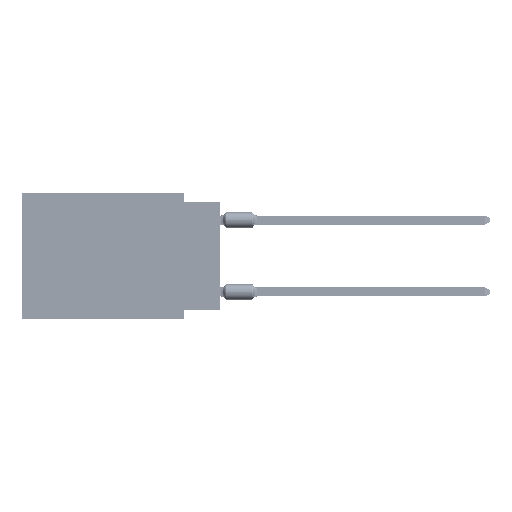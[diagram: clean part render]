
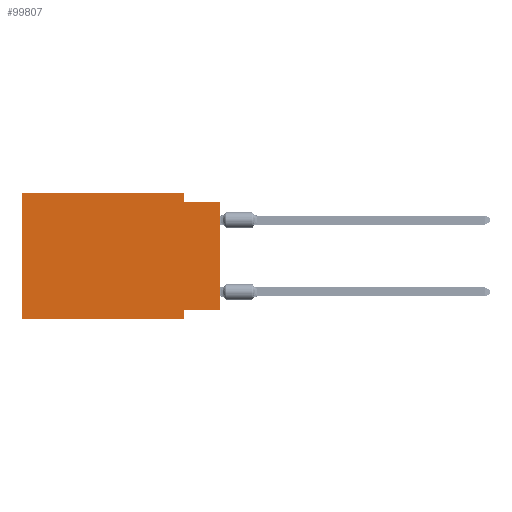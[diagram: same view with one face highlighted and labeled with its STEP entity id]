
A CAD part, left-side view. The second image highlights one B-rep face of the part: STEP entity #99807.
In plain terms, the highlighted planar face has unit normal (-1, 0, 0).
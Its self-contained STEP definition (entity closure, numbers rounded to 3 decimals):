
#3173 = VERTEX_POINT ( 'NONE', #75781 ) ;
#4792 = VERTEX_POINT ( 'NONE', #20576 ) ;
#7145 = EDGE_CURVE ( 'NONE', #107195, #94920, #32099, .T. ) ;
#7536 = AXIS2_PLACEMENT_3D ( 'NONE', #93989, #10364, #17118 ) ;
#9249 = VECTOR ( 'NONE', #37424, 1000. ) ;
#10364 = DIRECTION ( 'NONE',  ( 1., 0., 0. ) ) ;
#14214 = VECTOR ( 'NONE', #97078, 1000. ) ;
#14632 = CARTESIAN_POINT ( 'NONE',  ( 0., 0., -8.255 ) ) ;
#15207 = CARTESIAN_POINT ( 'NONE',  ( 0., 13.97, 0. ) ) ;
#15430 = EDGE_CURVE ( 'NONE', #4792, #97999, #85093, .T. ) ;
#17118 = DIRECTION ( 'NONE',  ( 0., 0., -1. ) ) ;
#20576 = CARTESIAN_POINT ( 'NONE',  ( 0., 2.54, 0. ) ) ;
#21849 = ORIENTED_EDGE ( 'NONE', *, *, #43082, .F. ) ;
#23670 = DIRECTION ( 'NONE',  ( 0., 0., 1. ) ) ;
#25764 = VECTOR ( 'NONE', #55518, 1000. ) ;
#26740 = LINE ( 'NONE', #52032, #101322 ) ;
#28451 = CARTESIAN_POINT ( 'NONE',  ( 0., 2.54, -8.89 ) ) ;
#30239 = CARTESIAN_POINT ( 'NONE',  ( 0., 13.97, 0. ) ) ;
#30744 = VERTEX_POINT ( 'NONE', #44216 ) ;
#32099 = LINE ( 'NONE', #66323, #98959 ) ;
#32378 = DIRECTION ( 'NONE',  ( 0., 0., -1. ) ) ;
#33443 = CARTESIAN_POINT ( 'NONE',  ( 0., 2.54, -8.255 ) ) ;
#37424 = DIRECTION ( 'NONE',  ( 0., 0., -1. ) ) ;
#38218 = DIRECTION ( 'NONE',  ( 0., 1., 0. ) ) ;
#38667 = LINE ( 'NONE', #30239, #25764 ) ;
#38704 = CARTESIAN_POINT ( 'NONE',  ( 0., 0., -8.255 ) ) ;
#40021 = EDGE_CURVE ( 'NONE', #107195, #47474, #65134, .T. ) ;
#41258 = EDGE_CURVE ( 'NONE', #3173, #30744, #57845, .T. ) ;
#43082 = EDGE_CURVE ( 'NONE', #47474, #57067, #45865, .T. ) ;
#44216 = CARTESIAN_POINT ( 'NONE',  ( 0., 13.97, 0. ) ) ;
#45865 = LINE ( 'NONE', #28451, #9249 ) ;
#46315 = ORIENTED_EDGE ( 'NONE', *, *, #101569, .F. ) ;
#47474 = VERTEX_POINT ( 'NONE', #33443 ) ;
#52032 = CARTESIAN_POINT ( 'NONE',  ( 0., 0., -0.635 ) ) ;
#53565 = PLANE ( 'NONE',  #7536 ) ;
#55518 = DIRECTION ( 'NONE',  ( 0., -1., 0. ) ) ;
#55679 = ORIENTED_EDGE ( 'NONE', *, *, #41258, .F. ) ;
#57067 = VERTEX_POINT ( 'NONE', #99077 ) ;
#57845 = LINE ( 'NONE', #15207, #62737 ) ;
#59766 = EDGE_CURVE ( 'NONE', #97999, #94920, #26740, .T. ) ;
#59873 = CARTESIAN_POINT ( 'NONE',  ( 0., 2.54, -0.635 ) ) ;
#62737 = VECTOR ( 'NONE', #90398, 1000. ) ;
#65134 = LINE ( 'NONE', #14632, #71224 ) ;
#66323 = CARTESIAN_POINT ( 'NONE',  ( 0., 0., 0. ) ) ;
#70733 = CARTESIAN_POINT ( 'NONE',  ( 0., 13.97, -8.89 ) ) ;
#71224 = VECTOR ( 'NONE', #38218, 1000. ) ;
#75044 = CARTESIAN_POINT ( 'NONE',  ( 0., 2.54, 0. ) ) ;
#75781 = CARTESIAN_POINT ( 'NONE',  ( 0., 13.97, -8.89 ) ) ;
#85093 = LINE ( 'NONE', #75044, #105151 ) ;
#87218 = FACE_OUTER_BOUND ( 'NONE', #100984, .T. ) ;
#90398 = DIRECTION ( 'NONE',  ( 0., 0., 1. ) ) ;
#93789 = LINE ( 'NONE', #70733, #14214 ) ;
#93989 = CARTESIAN_POINT ( 'NONE',  ( 0., 13.97, 0. ) ) ;
#94096 = DIRECTION ( 'NONE',  ( 0., -1., 0. ) ) ;
#94920 = VERTEX_POINT ( 'NONE', #95582 ) ;
#95582 = CARTESIAN_POINT ( 'NONE',  ( 0., 0., -0.635 ) ) ;
#97078 = DIRECTION ( 'NONE',  ( 0., -1., 0. ) ) ;
#97999 = VERTEX_POINT ( 'NONE', #59873 ) ;
#98959 = VECTOR ( 'NONE', #23670, 1000. ) ;
#99077 = CARTESIAN_POINT ( 'NONE',  ( 0., 2.54, -8.89 ) ) ;
#99807 = ADVANCED_FACE ( 'NONE', ( #87218 ), #53565, .F. ) ;
#100615 = ORIENTED_EDGE ( 'NONE', *, *, #108251, .T. ) ;
#100984 = EDGE_LOOP ( 'NONE', ( #106918, #106623, #105220, #46315, #55679, #100615, #21849, #106809 ) ) ;
#101322 = VECTOR ( 'NONE', #94096, 1000. ) ;
#101569 = EDGE_CURVE ( 'NONE', #30744, #4792, #38667, .T. ) ;
#105151 = VECTOR ( 'NONE', #32378, 1000. ) ;
#105220 = ORIENTED_EDGE ( 'NONE', *, *, #15430, .F. ) ;
#106623 = ORIENTED_EDGE ( 'NONE', *, *, #59766, .F. ) ;
#106809 = ORIENTED_EDGE ( 'NONE', *, *, #40021, .F. ) ;
#106918 = ORIENTED_EDGE ( 'NONE', *, *, #7145, .T. ) ;
#107195 = VERTEX_POINT ( 'NONE', #38704 ) ;
#108251 = EDGE_CURVE ( 'NONE', #3173, #57067, #93789, .T. ) ;
